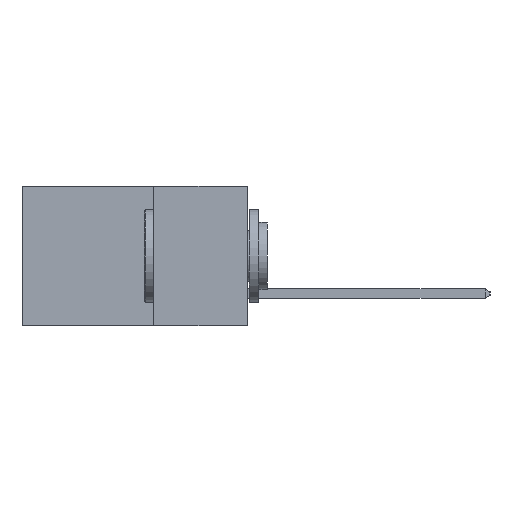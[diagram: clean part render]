
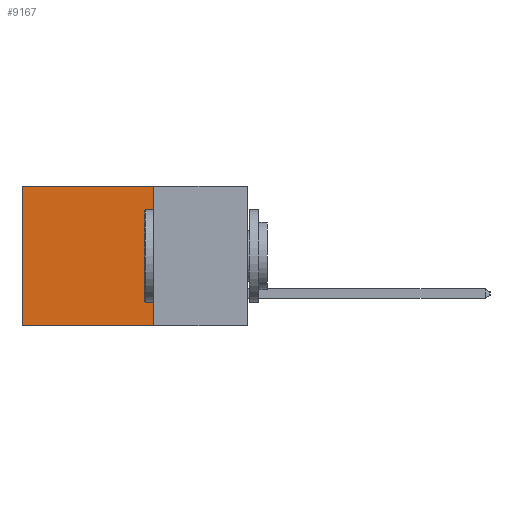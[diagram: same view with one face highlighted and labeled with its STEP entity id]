
A CAD part, left-side view. The second image highlights one B-rep face of the part: STEP entity #9167.
In plain terms, the highlighted planar face has unit normal (-1, 0, 0).
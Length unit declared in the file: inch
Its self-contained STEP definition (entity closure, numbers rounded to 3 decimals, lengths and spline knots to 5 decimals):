
#453 = LINE ( 'NONE', #10000, #4495 ) ;
#2692 = CARTESIAN_POINT ( 'NONE',  ( 0.298, 0.6, 0. ) ) ;
#2869 = EDGE_CURVE ( 'NONE', #16239, #11007, #9136, .T. ) ;
#2985 = EDGE_CURVE ( 'NONE', #16239, #11357, #21717, .T. ) ;
#3934 = CARTESIAN_POINT ( 'NONE',  ( 0.298, 0.25, -0.37 ) ) ;
#4495 = VECTOR ( 'NONE', #4819, 39.37008 ) ;
#4648 = DIRECTION ( 'NONE',  ( 0., 0., -1. ) ) ;
#4819 = DIRECTION ( 'NONE',  ( 0., 1., 0. ) ) ;
#4942 = DIRECTION ( 'NONE',  ( 0., 1., 0. ) ) ;
#5010 = EDGE_CURVE ( 'NONE', #11007, #21939, #453, .T. ) ;
#7701 = AXIS2_PLACEMENT_3D ( 'NONE', #24437, #23961, #23942 ) ;
#9136 = LINE ( 'NONE', #17265, #9710 ) ;
#9167 = ADVANCED_FACE ( 'NONE', ( #11571 ), #24039, .F. ) ;
#9179 = CARTESIAN_POINT ( 'NONE',  ( 0.298, 0.6, -0.37 ) ) ;
#9710 = VECTOR ( 'NONE', #24083, 39.37008 ) ;
#10000 = CARTESIAN_POINT ( 'NONE',  ( 0.298, 0.25, -0.37 ) ) ;
#11007 = VERTEX_POINT ( 'NONE', #3934 ) ;
#11175 = VECTOR ( 'NONE', #4942, 39.37008 ) ;
#11357 = VERTEX_POINT ( 'NONE', #15182 ) ;
#11571 = FACE_OUTER_BOUND ( 'NONE', #15893, .T. ) ;
#14806 = ORIENTED_EDGE ( 'NONE', *, *, #14882, .T. ) ;
#14882 = EDGE_CURVE ( 'NONE', #11357, #21939, #19158, .T. ) ;
#15182 = CARTESIAN_POINT ( 'NONE',  ( 0.298, 0.6, 0. ) ) ;
#15614 = ORIENTED_EDGE ( 'NONE', *, *, #2869, .F. ) ;
#15893 = EDGE_LOOP ( 'NONE', ( #14806, #17466, #15614, #16232 ) ) ;
#16232 = ORIENTED_EDGE ( 'NONE', *, *, #2985, .T. ) ;
#16239 = VERTEX_POINT ( 'NONE', #23699 ) ;
#17265 = CARTESIAN_POINT ( 'NONE',  ( 0.298, 0.25, 0. ) ) ;
#17466 = ORIENTED_EDGE ( 'NONE', *, *, #5010, .F. ) ;
#18566 = VECTOR ( 'NONE', #4648, 39.37008 ) ;
#19158 = LINE ( 'NONE', #2692, #18566 ) ;
#21717 = LINE ( 'NONE', #24462, #11175 ) ;
#21939 = VERTEX_POINT ( 'NONE', #9179 ) ;
#23699 = CARTESIAN_POINT ( 'NONE',  ( 0.298, 0.25, 0. ) ) ;
#23942 = DIRECTION ( 'NONE',  ( 0., 0., -1. ) ) ;
#23961 = DIRECTION ( 'NONE',  ( 1., 0., 0. ) ) ;
#24039 = PLANE ( 'NONE',  #7701 ) ;
#24083 = DIRECTION ( 'NONE',  ( 0., 0., -1. ) ) ;
#24437 = CARTESIAN_POINT ( 'NONE',  ( 0.298, 0.25, 0. ) ) ;
#24462 = CARTESIAN_POINT ( 'NONE',  ( 0.298, 0.25, 0. ) ) ;
